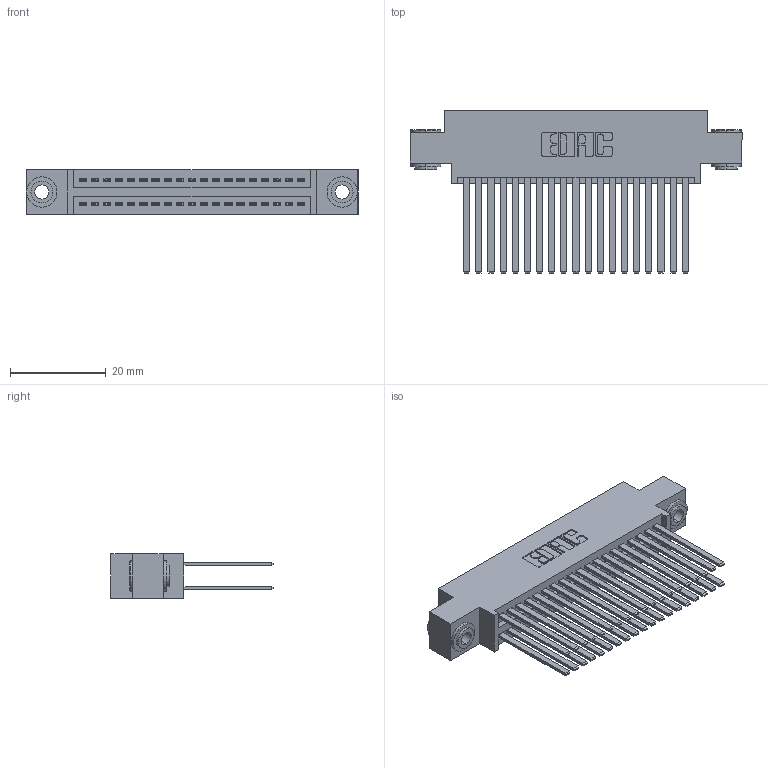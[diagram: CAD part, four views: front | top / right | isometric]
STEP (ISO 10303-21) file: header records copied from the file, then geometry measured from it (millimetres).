
FILE_DESCRIPTION (( 'STEP AP203' ), '1' );
FILE_NAME ('345-038-544-803.STEP', '2019-10-28T15:34:42', ( '' ), ( '' ), 'SwSTEP 2.0', 'SolidWorks 2016', '' );
FILE_SCHEMA (( 'CONFIG_CONTROL_DESIGN' ));
Length unit declared in the file: inch
Products named in the file (4): 345-250-002_345-250-002-102; 345 Part_0.170 Offset - 0.156 Dia-TH; 345-038-544-803; 345-292-001_345-293-144
Assembly tree (41 placements, depth 2):
  345-038-544-803
    345 Part_0.170 Offset - 0.156 Dia-TH
    345-292-001_345-293-144  x38
    345-250-002_345-250-002-102  x2
Bounding box: 69.47 x 33.96 x 9.4 mm (x, y, z)
Volume: 6973.5 mm3; surface area: 11772.2 mm2
Topology: 41 solids, 41 shells, 1840 faces, 5407 edges, 3550 vertices
Faces by surface type: plane 1196, cylinder 636, cone 8
Entity records: 18602 total; most frequent: CARTESIAN_POINT 3115, ORIENTED_EDGE 3042, DIRECTION 2803, EDGE_CURVE 1521, VECTOR 1293, LINE 1293, VERTEX_POINT 1010, AXIS2_PLACEMENT_3D 755
